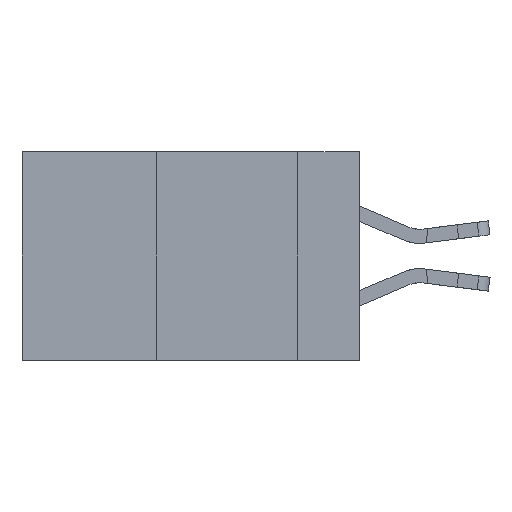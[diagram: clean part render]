
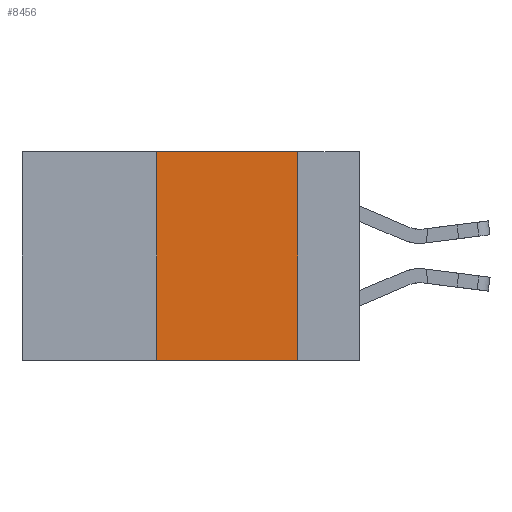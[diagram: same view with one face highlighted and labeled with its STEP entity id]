
A CAD part, left-side view. The second image highlights one B-rep face of the part: STEP entity #8456.
In plain terms, the highlighted planar face has unit normal (-1, 0, 0).
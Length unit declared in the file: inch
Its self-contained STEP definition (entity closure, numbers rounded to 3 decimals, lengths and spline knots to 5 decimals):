
#113 = CARTESIAN_POINT ( 'NONE',  ( 0., 0.36, 0. ) ) ;
#1254 = ORIENTED_EDGE ( 'NONE', *, *, #4413, .F. ) ;
#1375 = FACE_OUTER_BOUND ( 'NONE', #11265, .T. ) ;
#2343 = CARTESIAN_POINT ( 'NONE',  ( 0., 0.6, -0.37 ) ) ;
#2902 = EDGE_CURVE ( 'NONE', #8734, #15755, #17121, .T. ) ;
#4413 = EDGE_CURVE ( 'NONE', #17664, #8734, #5561, .T. ) ;
#5434 = EDGE_CURVE ( 'NONE', #14774, #15755, #6412, .T. ) ;
#5545 = CARTESIAN_POINT ( 'NONE',  ( 0., 0.36, 0. ) ) ;
#5561 = LINE ( 'NONE', #16042, #6681 ) ;
#6412 = LINE ( 'NONE', #2343, #19110 ) ;
#6681 = VECTOR ( 'NONE', #7197, 39.37008 ) ;
#6810 = VECTOR ( 'NONE', #15292, 39.37008 ) ;
#7197 = DIRECTION ( 'NONE',  ( 0., -1., 0. ) ) ;
#8446 = LINE ( 'NONE', #5545, #6810 ) ;
#8456 = ADVANCED_FACE ( 'NONE', ( #1375 ), #18115, .F. ) ;
#8734 = VERTEX_POINT ( 'NONE', #11266 ) ;
#9592 = DIRECTION ( 'NONE',  ( 0., -1., 0. ) ) ;
#10086 = ORIENTED_EDGE ( 'NONE', *, *, #11614, .F. ) ;
#10412 = CARTESIAN_POINT ( 'NONE',  ( 0., 0.11, 0. ) ) ;
#11145 = VECTOR ( 'NONE', #17674, 39.37008 ) ;
#11265 = EDGE_LOOP ( 'NONE', ( #17946, #1254, #10086, #13631 ) ) ;
#11266 = CARTESIAN_POINT ( 'NONE',  ( 0., 0.11, 0. ) ) ;
#11614 = EDGE_CURVE ( 'NONE', #14774, #17664, #8446, .T. ) ;
#13631 = ORIENTED_EDGE ( 'NONE', *, *, #5434, .T. ) ;
#14245 = DIRECTION ( 'NONE',  ( 1., 0., 0. ) ) ;
#14774 = VERTEX_POINT ( 'NONE', #17526 ) ;
#14835 = CARTESIAN_POINT ( 'NONE',  ( 0., 0.11, -0.37 ) ) ;
#15166 = CARTESIAN_POINT ( 'NONE',  ( 0., 0.6, 0. ) ) ;
#15292 = DIRECTION ( 'NONE',  ( 0., 0., 1. ) ) ;
#15755 = VERTEX_POINT ( 'NONE', #14835 ) ;
#15891 = DIRECTION ( 'NONE',  ( 0., 0., -1. ) ) ;
#16042 = CARTESIAN_POINT ( 'NONE',  ( 0., 0.6, 0. ) ) ;
#17121 = LINE ( 'NONE', #10412, #11145 ) ;
#17526 = CARTESIAN_POINT ( 'NONE',  ( 0., 0.36, -0.37 ) ) ;
#17664 = VERTEX_POINT ( 'NONE', #113 ) ;
#17674 = DIRECTION ( 'NONE',  ( 0., 0., -1. ) ) ;
#17938 = AXIS2_PLACEMENT_3D ( 'NONE', #15166, #14245, #15891 ) ;
#17946 = ORIENTED_EDGE ( 'NONE', *, *, #2902, .F. ) ;
#18115 = PLANE ( 'NONE',  #17938 ) ;
#19110 = VECTOR ( 'NONE', #9592, 39.37008 ) ;
